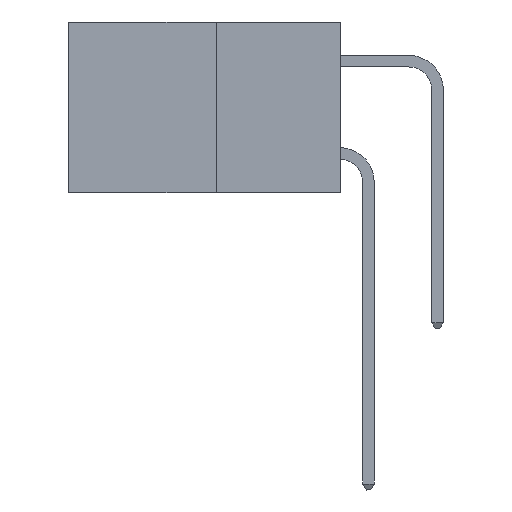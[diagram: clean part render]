
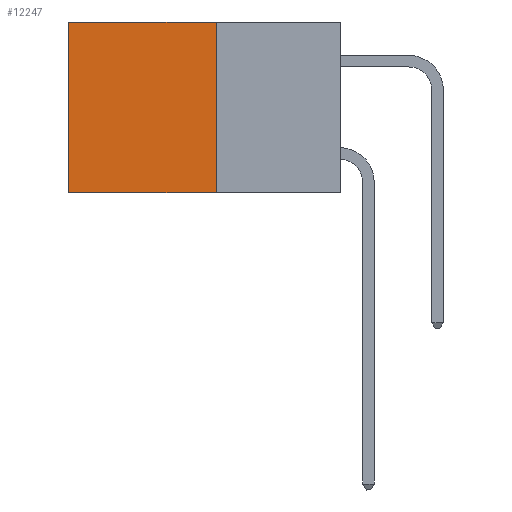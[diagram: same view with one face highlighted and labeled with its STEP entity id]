
A CAD part, left-side view. The second image highlights one B-rep face of the part: STEP entity #12247.
In plain terms, the highlighted planar face has unit normal (-1, 0, 0).
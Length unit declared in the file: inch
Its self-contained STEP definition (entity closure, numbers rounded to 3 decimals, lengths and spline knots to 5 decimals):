
#107 = DIRECTION ( 'NONE',  ( 0., 0., -1. ) ) ;
#1101 = LINE ( 'NONE', #11169, #14284 ) ;
#1414 = LINE ( 'NONE', #9521, #6432 ) ;
#2349 = EDGE_LOOP ( 'NONE', ( #19564, #18442, #18762, #14253 ) ) ;
#2763 = DIRECTION ( 'NONE',  ( 0., 0., -1. ) ) ;
#3672 = EDGE_CURVE ( 'NONE', #19224, #16192, #22165, .T. ) ;
#4558 = CARTESIAN_POINT ( 'NONE',  ( 0.277, 0.27, -0.37 ) ) ;
#4771 = DIRECTION ( 'NONE',  ( 0., 1., 0. ) ) ;
#4871 = CARTESIAN_POINT ( 'NONE',  ( 0.277, 0.27, -0.37 ) ) ;
#5021 = CARTESIAN_POINT ( 'NONE',  ( 0.277, 0.59, -0.37 ) ) ;
#6432 = VECTOR ( 'NONE', #20733, 39.37008 ) ;
#7264 = VECTOR ( 'NONE', #2763, 39.37008 ) ;
#8483 = VERTEX_POINT ( 'NONE', #5021 ) ;
#9521 = CARTESIAN_POINT ( 'NONE',  ( 0.277, 0.59, -0.37 ) ) ;
#10260 = CARTESIAN_POINT ( 'NONE',  ( 0.277, 0.27, 0. ) ) ;
#11086 = EDGE_CURVE ( 'NONE', #17460, #8483, #1414, .T. ) ;
#11169 = CARTESIAN_POINT ( 'NONE',  ( 0.277, 0.27, -0.37 ) ) ;
#11330 = DIRECTION ( 'NONE',  ( 1., 0., 0. ) ) ;
#11946 = CARTESIAN_POINT ( 'NONE',  ( 0.277, 0.59, 0. ) ) ;
#12247 = ADVANCED_FACE ( 'NONE', ( #15398 ), #22523, .F. ) ;
#13025 = DIRECTION ( 'NONE',  ( 0., 1., 0. ) ) ;
#14042 = AXIS2_PLACEMENT_3D ( 'NONE', #20508, #11330, #107 ) ;
#14253 = ORIENTED_EDGE ( 'NONE', *, *, #21415, .T. ) ;
#14284 = VECTOR ( 'NONE', #13025, 39.37008 ) ;
#15398 = FACE_OUTER_BOUND ( 'NONE', #2349, .T. ) ;
#16192 = VERTEX_POINT ( 'NONE', #4558 ) ;
#17152 = EDGE_CURVE ( 'NONE', #16192, #8483, #1101, .T. ) ;
#17238 = VECTOR ( 'NONE', #4771, 39.37008 ) ;
#17460 = VERTEX_POINT ( 'NONE', #11946 ) ;
#17820 = LINE ( 'NONE', #10260, #17238 ) ;
#18442 = ORIENTED_EDGE ( 'NONE', *, *, #17152, .F. ) ;
#18762 = ORIENTED_EDGE ( 'NONE', *, *, #3672, .F. ) ;
#19224 = VERTEX_POINT ( 'NONE', #19611 ) ;
#19564 = ORIENTED_EDGE ( 'NONE', *, *, #11086, .T. ) ;
#19611 = CARTESIAN_POINT ( 'NONE',  ( 0.277, 0.27, 0. ) ) ;
#20508 = CARTESIAN_POINT ( 'NONE',  ( 0.277, 0.27, -0.37 ) ) ;
#20733 = DIRECTION ( 'NONE',  ( 0., 0., -1. ) ) ;
#21415 = EDGE_CURVE ( 'NONE', #19224, #17460, #17820, .T. ) ;
#22165 = LINE ( 'NONE', #4871, #7264 ) ;
#22523 = PLANE ( 'NONE',  #14042 ) ;
